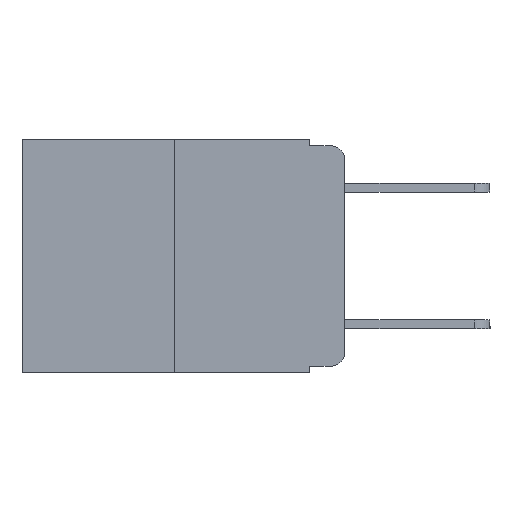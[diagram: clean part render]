
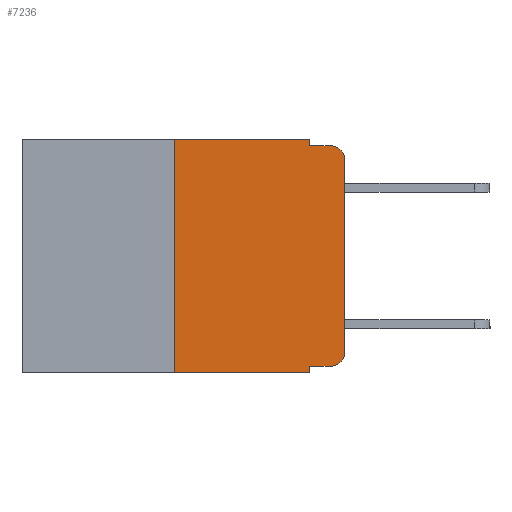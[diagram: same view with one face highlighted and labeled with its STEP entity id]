
A CAD part, left-side view. The second image highlights one B-rep face of the part: STEP entity #7236.
In plain terms, the highlighted planar face has unit normal (-1, 0, 0).
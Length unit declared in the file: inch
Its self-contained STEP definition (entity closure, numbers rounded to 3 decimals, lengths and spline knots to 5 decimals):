
#57 = EDGE_CURVE ( 'NONE', #9363, #6201, #11583, .T. ) ;
#60 = VERTEX_POINT ( 'NONE', #6441 ) ;
#89 = DIRECTION ( 'NONE',  ( 0., 0., -1. ) ) ;
#141 = EDGE_CURVE ( 'NONE', #9323, #5366, #399, .T. ) ;
#304 = AXIS2_PLACEMENT_3D ( 'NONE', #10083, #11091, #89 ) ;
#399 = LINE ( 'NONE', #4441, #4886 ) ;
#753 = EDGE_LOOP ( 'NONE', ( #4325, #3207, #4011, #6436, #12529, #1346, #12348, #1317, #11587, #6789 ) ) ;
#833 = LINE ( 'NONE', #1037, #4152 ) ;
#1037 = CARTESIAN_POINT ( 'NONE',  ( 0., 0.051, 0. ) ) ;
#1185 = EDGE_CURVE ( 'NONE', #5838, #4881, #4190, .T. ) ;
#1317 = ORIENTED_EDGE ( 'NONE', *, *, #11150, .F. ) ;
#1346 = ORIENTED_EDGE ( 'NONE', *, *, #11138, .F. ) ;
#1973 = DIRECTION ( 'NONE',  ( 0., 0., -1. ) ) ;
#2000 = DIRECTION ( 'NONE',  ( 0., -1., 0. ) ) ;
#2137 = LINE ( 'NONE', #5153, #6294 ) ;
#2593 = VERTEX_POINT ( 'NONE', #7145 ) ;
#2774 = DIRECTION ( 'NONE',  ( -1., 0., 0. ) ) ;
#3207 = ORIENTED_EDGE ( 'NONE', *, *, #11858, .T. ) ;
#3240 = EDGE_CURVE ( 'NONE', #60, #7496, #11695, .T. ) ;
#3502 = PLANE ( 'NONE',  #9052 ) ;
#3504 = VECTOR ( 'NONE', #8509, 39.37008 ) ;
#3600 = VERTEX_POINT ( 'NONE', #4677 ) ;
#3764 = DIRECTION ( 'NONE',  ( 0., 0., -1. ) ) ;
#4011 = ORIENTED_EDGE ( 'NONE', *, *, #141, .F. ) ;
#4152 = VECTOR ( 'NONE', #1973, 39.37008 ) ;
#4190 = LINE ( 'NONE', #6321, #4625 ) ;
#4325 = ORIENTED_EDGE ( 'NONE', *, *, #12359, .T. ) ;
#4360 = VECTOR ( 'NONE', #12387, 39.37008 ) ;
#4441 = CARTESIAN_POINT ( 'NONE',  ( 0., 0.051, -0.01 ) ) ;
#4559 = CARTESIAN_POINT ( 'NONE',  ( 0., 0.473, 0. ) ) ;
#4625 = VECTOR ( 'NONE', #8315, 39.37008 ) ;
#4677 = CARTESIAN_POINT ( 'NONE',  ( 0., 0., -0.03 ) ) ;
#4881 = VERTEX_POINT ( 'NONE', #5155 ) ;
#4886 = VECTOR ( 'NONE', #5773, 39.37008 ) ;
#5153 = CARTESIAN_POINT ( 'NONE',  ( 0., 0.051, -0.333 ) ) ;
#5155 = CARTESIAN_POINT ( 'NONE',  ( 0., 0.051, -0.343 ) ) ;
#5299 = AXIS2_PLACEMENT_3D ( 'NONE', #11179, #2774, #3764 ) ;
#5366 = VERTEX_POINT ( 'NONE', #11734 ) ;
#5368 = CARTESIAN_POINT ( 'NONE',  ( 0., 0., -0.313 ) ) ;
#5773 = DIRECTION ( 'NONE',  ( 0., -1., 0. ) ) ;
#5838 = VERTEX_POINT ( 'NONE', #12783 ) ;
#6201 = VERTEX_POINT ( 'NONE', #7473 ) ;
#6294 = VECTOR ( 'NONE', #2000, 39.37008 ) ;
#6321 = CARTESIAN_POINT ( 'NONE',  ( 0., 0.473, -0.343 ) ) ;
#6436 = ORIENTED_EDGE ( 'NONE', *, *, #9319, .F. ) ;
#6441 = CARTESIAN_POINT ( 'NONE',  ( 0., 0.02, -0.333 ) ) ;
#6559 = DIRECTION ( 'NONE',  ( 0., 0., 1. ) ) ;
#6789 = ORIENTED_EDGE ( 'NONE', *, *, #3240, .T. ) ;
#6994 = CARTESIAN_POINT ( 'NONE',  ( 0., 0.25, 0. ) ) ;
#7145 = CARTESIAN_POINT ( 'NONE',  ( 0., 0.051, -0.333 ) ) ;
#7236 = ADVANCED_FACE ( 'NONE', ( #9583 ), #3502, .F. ) ;
#7377 = CARTESIAN_POINT ( 'NONE',  ( 0., 0.051, 0. ) ) ;
#7438 = VECTOR ( 'NONE', #12591, 39.37008 ) ;
#7473 = CARTESIAN_POINT ( 'NONE',  ( 0., 0.051, 0. ) ) ;
#7496 = VERTEX_POINT ( 'NONE', #5368 ) ;
#8309 = LINE ( 'NONE', #7377, #4360 ) ;
#8315 = DIRECTION ( 'NONE',  ( 0., -1., 0. ) ) ;
#8509 = DIRECTION ( 'NONE',  ( 0., 0., 1. ) ) ;
#8568 = DIRECTION ( 'NONE',  ( 0., 0., -1. ) ) ;
#8871 = VECTOR ( 'NONE', #6559, 39.37008 ) ;
#9052 = AXIS2_PLACEMENT_3D ( 'NONE', #10720, #11522, #8568 ) ;
#9319 = EDGE_CURVE ( 'NONE', #6201, #9323, #833, .T. ) ;
#9323 = VERTEX_POINT ( 'NONE', #11140 ) ;
#9363 = VERTEX_POINT ( 'NONE', #6994 ) ;
#9583 = FACE_OUTER_BOUND ( 'NONE', #753, .T. ) ;
#9623 = LINE ( 'NONE', #9826, #8871 ) ;
#9826 = CARTESIAN_POINT ( 'NONE',  ( 0., 0., 0. ) ) ;
#10083 = CARTESIAN_POINT ( 'NONE',  ( 0., 0.02, -0.03 ) ) ;
#10720 = CARTESIAN_POINT ( 'NONE',  ( 0., 0.473, 0. ) ) ;
#11091 = DIRECTION ( 'NONE',  ( -1., 0., 0. ) ) ;
#11138 = EDGE_CURVE ( 'NONE', #5838, #9363, #11517, .T. ) ;
#11140 = CARTESIAN_POINT ( 'NONE',  ( 0., 0.051, -0.01 ) ) ;
#11150 = EDGE_CURVE ( 'NONE', #2593, #4881, #8309, .T. ) ;
#11179 = CARTESIAN_POINT ( 'NONE',  ( 0., 0.02, -0.313 ) ) ;
#11384 = EDGE_CURVE ( 'NONE', #2593, #60, #2137, .T. ) ;
#11393 = CARTESIAN_POINT ( 'NONE',  ( 0., 0.25, 0. ) ) ;
#11517 = LINE ( 'NONE', #11393, #3504 ) ;
#11522 = DIRECTION ( 'NONE',  ( 1., 0., 0. ) ) ;
#11583 = LINE ( 'NONE', #4559, #7438 ) ;
#11587 = ORIENTED_EDGE ( 'NONE', *, *, #11384, .T. ) ;
#11695 = CIRCLE ( 'NONE', #5299, 0.02 ) ;
#11734 = CARTESIAN_POINT ( 'NONE',  ( 0., 0.02, -0.01 ) ) ;
#11858 = EDGE_CURVE ( 'NONE', #3600, #5366, #12278, .T. ) ;
#12278 = CIRCLE ( 'NONE', #304, 0.02 ) ;
#12348 = ORIENTED_EDGE ( 'NONE', *, *, #1185, .T. ) ;
#12359 = EDGE_CURVE ( 'NONE', #7496, #3600, #9623, .T. ) ;
#12387 = DIRECTION ( 'NONE',  ( 0., 0., -1. ) ) ;
#12529 = ORIENTED_EDGE ( 'NONE', *, *, #57, .F. ) ;
#12591 = DIRECTION ( 'NONE',  ( 0., -1., 0. ) ) ;
#12783 = CARTESIAN_POINT ( 'NONE',  ( 0., 0.25, -0.343 ) ) ;
